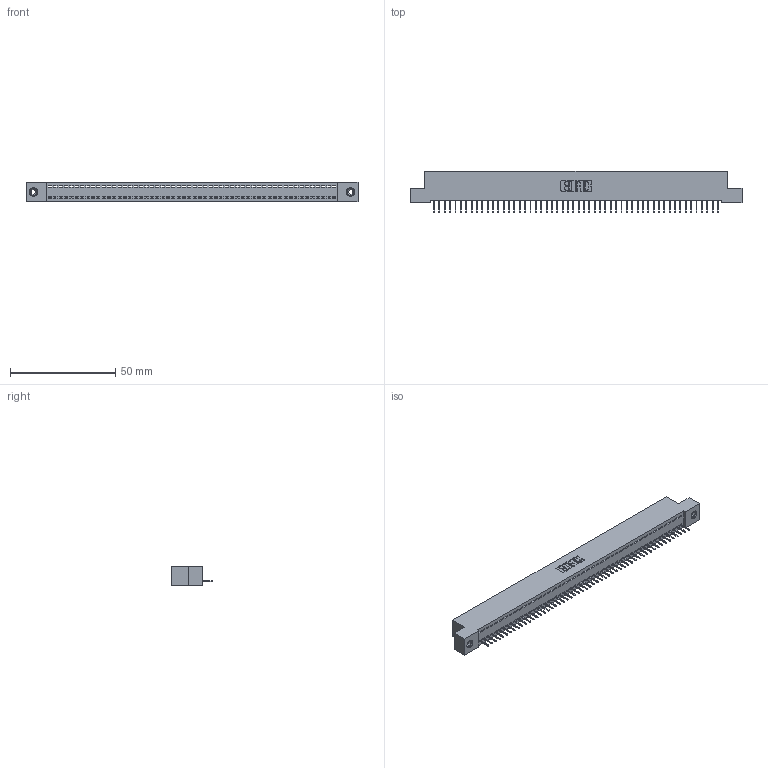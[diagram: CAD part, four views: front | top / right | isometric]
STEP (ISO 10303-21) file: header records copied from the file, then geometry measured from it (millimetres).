
FILE_DESCRIPTION (( 'STEP AP203' ), '1' );
FILE_NAME ('392-054-524-108.STEP', '2018-08-17T08:43:05', ( '' ), ( '' ), 'SwSTEP 2.0', 'SolidWorks 2016', '' );
FILE_SCHEMA (( 'CONFIG_CONTROL_DESIGN' ));
Length unit declared in the file: inch
Products named in the file (4): 345-250-001_345-250-003-102; 392-054-524-108; 342 Part_TI; 345-292-001_345-293-124
Assembly tree (57 placements, depth 2):
  392-054-524-108
    342 Part_TI
    345-292-001_345-293-124  x54
    345-250-001_345-250-003-102  x2
Bounding box: 157.48 x 19.69 x 9.4 mm (x, y, z)
Volume: 13633.1 mm3; surface area: 19598.8 mm2
Topology: 57 solids, 57 shells, 3518 faces, 10155 edges, 6546 vertices
Faces by surface type: plane 2690, cylinder 812, cone 12, torus 4
Entity records: 32588 total; most frequent: CARTESIAN_POINT 5599, ORIENTED_EDGE 5582, DIRECTION 4733, EDGE_CURVE 2791, LINE 2647, VECTOR 2647, VERTEX_POINT 1852, AXIS2_PLACEMENT_3D 1043
